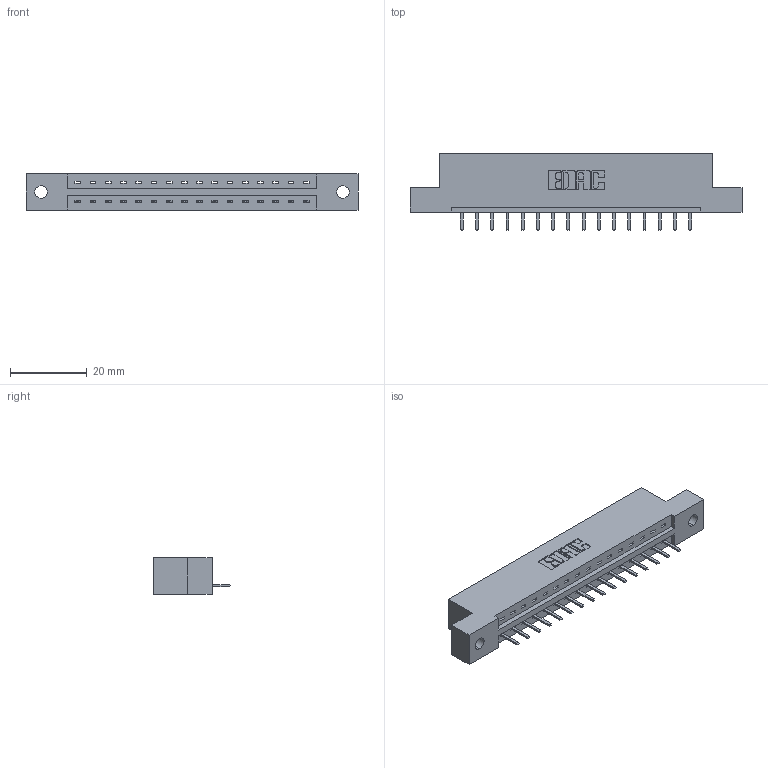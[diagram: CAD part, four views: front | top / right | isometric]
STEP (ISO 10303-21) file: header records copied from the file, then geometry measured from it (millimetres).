
FILE_DESCRIPTION (( 'STEP AP203' ), '1' );
FILE_NAME ('387-016-520-102.STEP', '2019-10-02T17:55:54', ( '' ), ( '' ), 'SwSTEP 2.0', 'SolidWorks 2016', '' );
FILE_SCHEMA (( 'CONFIG_CONTROL_DESIGN' ));
Length unit declared in the file: inch
Products named in the file (3): 387-016-520-102; 345-292-001_345-293-120; 337 Part_Flush Mounting Lugs - 0.128 Dia
Assembly tree (17 placements, depth 2):
  387-016-520-102
    337 Part_Flush Mounting Lugs - 0.128 Dia
    345-292-001_345-293-120  x16
Bounding box: 86.41 x 20.02 x 9.4 mm (x, y, z)
Volume: 8572.9 mm3; surface area: 8279 mm2
Topology: 17 solids, 17 shells, 1170 faces, 3447 edges, 2254 vertices
Faces by surface type: plane 838, cylinder 332
Entity records: 15373 total; most frequent: CARTESIAN_POINT 2694, ORIENTED_EDGE 2634, DIRECTION 2309, EDGE_CURVE 1317, VECTOR 1185, LINE 1185, VERTEX_POINT 874, AXIS2_PLACEMENT_3D 562
